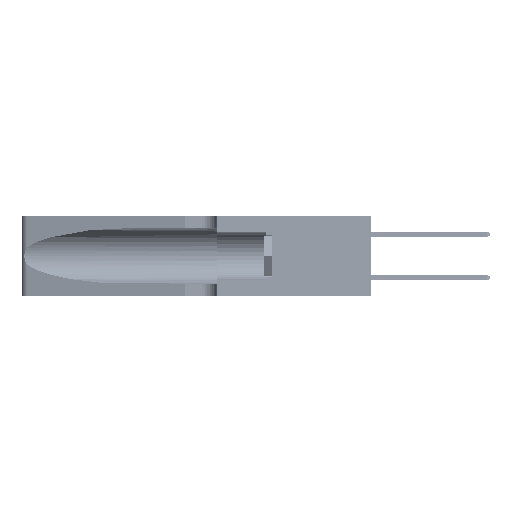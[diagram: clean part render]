
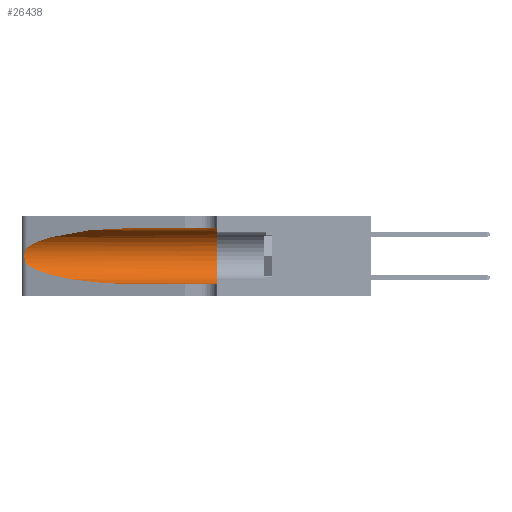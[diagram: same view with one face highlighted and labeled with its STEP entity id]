
A CAD part, left-side view. The second image highlights one B-rep face of the part: STEP entity #26438.
In plain terms, the highlighted cylindrical face has radius 3.308 mm (diameter 6.617 mm), a partial arc.
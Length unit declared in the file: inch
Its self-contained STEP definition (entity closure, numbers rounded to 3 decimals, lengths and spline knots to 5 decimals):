
#48 = EDGE_CURVE ( 'NONE', #10058, #5362, #40471, .T. ) ;
#295 = ORIENTED_EDGE ( 'NONE', *, *, #35026, .T. ) ;
#568 = VERTEX_POINT ( 'NONE', #36704 ) ;
#698 = LINE ( 'NONE', #12758, #8994 ) ;
#1474 = CARTESIAN_POINT ( 'NONE',  ( 0.25487, 1.22718, 0.14631 ) ) ;
#4835 = CARTESIAN_POINT ( 'NONE',  ( 0.25787, 1.23484, 0.2124 ) ) ;
#5356 = CARTESIAN_POINT ( 'NONE',  ( 0.1305, 0.72297, 0.05475 ) ) ;
#5362 = VERTEX_POINT ( 'NONE', #29737 ) ;
#6071 = VERTEX_POINT ( 'NONE', #1474 ) ;
#6331 = VERTEX_POINT ( 'NONE', #35569 ) ;
#8468 = LINE ( 'NONE', #14566, #18042 ) ;
#8770 = CARTESIAN_POINT ( 'NONE',  ( 0.25555, 1.22994, 0.2215 ) ) ;
#8955 = CARTESIAN_POINT ( 'NONE',  ( 0.26018, 1.23835, 0.19895 ) ) ;
#8994 = VECTOR ( 'NONE', #16840, 39.37008 ) ;
#9753 = AXIS2_PLACEMENT_3D ( 'NONE', #35036, #26806, #10541 ) ;
#10058 = VERTEX_POINT ( 'NONE', #15100 ) ;
#10541 = DIRECTION ( 'NONE',  ( 0., 0., -1. ) ) ;
#11064 = CARTESIAN_POINT ( 'NONE',  ( 0.1305, 0.72297, 0.31525 ) ) ;
#12378 = CYLINDRICAL_SURFACE ( 'NONE', #9753, 0.13025 ) ;
#12758 = CARTESIAN_POINT ( 'NONE',  ( 0.1305, 1.61858, 0.05475 ) ) ;
#12940 = DIRECTION ( 'NONE',  ( 0., 1., 0. ) ) ;
#13048 = CARTESIAN_POINT ( 'NONE',  ( 0.26075, 1.23896, 0.178 ) ) ;
#14523 = B_SPLINE_CURVE_WITH_KNOTS ( 'NONE', 3,
 ( #49644, #8770, #29292, #4835, #33417, #8955, #37537, #13048, #41644, #17137, #45741, #21272, #49819, #25366 ),
 .UNSPECIFIED., .F., .F.,
 ( 4, 2, 2, 2, 2, 2, 4 ),
 ( 0., 0.00027, 0.00053, 0.00107, 0.0016, 0.00187, 0.00214 ),
 .UNSPECIFIED. ) ;
#14566 = CARTESIAN_POINT ( 'NONE',  ( 0.1305, 1.61858, 0.31525 ) ) ;
#15100 = CARTESIAN_POINT ( 'NONE',  ( 0.1305, 0.35, 0.31525 ) ) ;
#15161 = CARTESIAN_POINT ( 'NONE',  ( 0.2373, 1.15595, 0.28018 ) ) ;
#15546 = ORIENTED_EDGE ( 'NONE', *, *, #38710, .F. ) ;
#16840 = DIRECTION ( 'NONE',  ( 0., -1., 0. ) ) ;
#17137 = CARTESIAN_POINT ( 'NONE',  ( 0.25856, 1.23593, 0.16098 ) ) ;
#17461 = CARTESIAN_POINT ( 'NONE',  ( 0.1305, 0.72297, 0.05475 ) ) ;
#18042 = VECTOR ( 'NONE', #34950, 39.37008 ) ;
#20351 = ORIENTED_EDGE ( 'NONE', *, *, #46379, .T. ) ;
#21272 = CARTESIAN_POINT ( 'NONE',  ( 0.25639, 1.23186, 0.15144 ) ) ;
#25366 = CARTESIAN_POINT ( 'NONE',  ( 0.25487, 1.22718, 0.14631 ) ) ;
#25880 = ORIENTED_EDGE ( 'NONE', *, *, #49901, .T. ) ;
#26438 = ADVANCED_FACE ( 'NONE', ( #34130 ), #12378, .F. ) ;
#26806 = DIRECTION ( 'NONE',  ( 0., -1., 0. ) ) ;
#27028 = ORIENTED_EDGE ( 'NONE', *, *, #50869, .T. ) ;
#29292 = CARTESIAN_POINT ( 'NONE',  ( 0.25639, 1.23184, 0.21858 ) ) ;
#29737 = CARTESIAN_POINT ( 'NONE',  ( 0.1305, 0.35, 0.05475 ) ) ;
#29830 = CARTESIAN_POINT ( 'NONE',  ( 0.18966, 0.96281, 0.05475 ) ) ;
#30039 = VERTEX_POINT ( 'NONE', #17461 ) ;
#31224 =( BOUNDED_CURVE ( )  B_SPLINE_CURVE ( 3, ( #42002, #46091, #29830, #5356 ),
 .UNSPECIFIED., .F., .F. ) 
 B_SPLINE_CURVE_WITH_KNOTS ( ( 4, 4 ),
 ( 3.44316, 4.71239 ),
 .UNSPECIFIED. ) 
 CURVE ( )  GEOMETRIC_REPRESENTATION_ITEM ( )  RATIONAL_B_SPLINE_CURVE ( ( 1., 0.87, 0.87, 1. ) ) 
 REPRESENTATION_ITEM ( '' )  );
#31592 = AXIS2_PLACEMENT_3D ( 'NONE', #37423, #12940, #41542 ) ;
#33417 = CARTESIAN_POINT ( 'NONE',  ( 0.25854, 1.2359, 0.20912 ) ) ;
#34030 = EDGE_LOOP ( 'NONE', ( #25880, #295, #20351, #27028, #43817, #15546 ) ) ;
#34130 = FACE_OUTER_BOUND ( 'NONE', #34030, .T. ) ;
#34950 = DIRECTION ( 'NONE',  ( 0., -1., 0. ) ) ;
#35026 = EDGE_CURVE ( 'NONE', #568, #6071, #14523, .T. ) ;
#35036 = CARTESIAN_POINT ( 'NONE',  ( 0.1305, 1.61858, 0.185 ) ) ;
#35569 = CARTESIAN_POINT ( 'NONE',  ( 0.1305, 0.72297, 0.31525 ) ) ;
#36704 = CARTESIAN_POINT ( 'NONE',  ( 0.25487, 1.22718, 0.22369 ) ) ;
#37423 = CARTESIAN_POINT ( 'NONE',  ( 0.1305, 0.35, 0.185 ) ) ;
#37537 = CARTESIAN_POINT ( 'NONE',  ( 0.26075, 1.23896, 0.19203 ) ) ;
#38710 = EDGE_CURVE ( 'NONE', #6331, #10058, #8468, .T. ) ;
#40471 = CIRCLE ( 'NONE', #31592, 0.13025 ) ;
#41542 = DIRECTION ( 'NONE',  ( 0., 0., 1. ) ) ;
#41644 = CARTESIAN_POINT ( 'NONE',  ( 0.26017, 1.23833, 0.17102 ) ) ;
#42002 = CARTESIAN_POINT ( 'NONE',  ( 0.25487, 1.22718, 0.14631 ) ) ;
#43748 = CARTESIAN_POINT ( 'NONE',  ( 0.25487, 1.22718, 0.22369 ) ) ;
#43817 = ORIENTED_EDGE ( 'NONE', *, *, #48, .F. ) ;
#45741 = CARTESIAN_POINT ( 'NONE',  ( 0.25789, 1.23486, 0.15765 ) ) ;
#46091 = CARTESIAN_POINT ( 'NONE',  ( 0.2373, 1.15595, 0.08982 ) ) ;
#46379 = EDGE_CURVE ( 'NONE', #6071, #30039, #31224, .T. ) ;
#47652 = CARTESIAN_POINT ( 'NONE',  ( 0.18966, 0.96281, 0.31525 ) ) ;
#49644 = CARTESIAN_POINT ( 'NONE',  ( 0.25487, 1.22718, 0.22369 ) ) ;
#49819 = CARTESIAN_POINT ( 'NONE',  ( 0.25555, 1.22993, 0.14849 ) ) ;
#49901 = EDGE_CURVE ( 'NONE', #6331, #568, #50183, .T. ) ;
#50183 =( BOUNDED_CURVE ( )  B_SPLINE_CURVE ( 3, ( #11064, #47652, #15161, #43748 ),
 .UNSPECIFIED., .F., .F. ) 
 B_SPLINE_CURVE_WITH_KNOTS ( ( 4, 4 ),
 ( 1.5708, 2.84003 ),
 .UNSPECIFIED. ) 
 CURVE ( )  GEOMETRIC_REPRESENTATION_ITEM ( )  RATIONAL_B_SPLINE_CURVE ( ( 1., 0.87, 0.87, 1. ) ) 
 REPRESENTATION_ITEM ( '' )  );
#50869 = EDGE_CURVE ( 'NONE', #30039, #5362, #698, .T. ) ;
